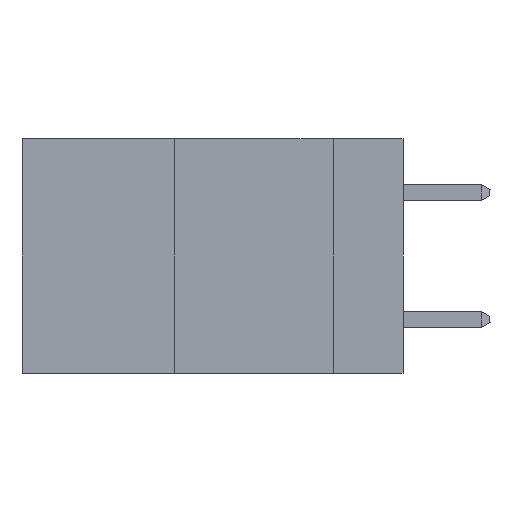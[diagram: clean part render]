
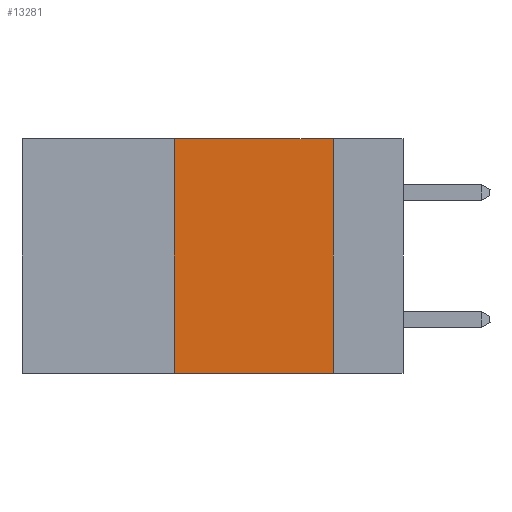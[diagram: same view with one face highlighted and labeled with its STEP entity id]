
A CAD part, left-side view. The second image highlights one B-rep face of the part: STEP entity #13281.
In plain terms, the highlighted planar face has unit normal (-1, 0, 0).
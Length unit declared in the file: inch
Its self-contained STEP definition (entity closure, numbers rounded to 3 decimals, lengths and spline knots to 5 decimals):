
#2290 = DIRECTION ( 'NONE',  ( 0., 0., -1. ) ) ;
#2624 = VECTOR ( 'NONE', #29477, 39.37008 ) ;
#3059 = EDGE_CURVE ( 'NONE', #30316, #32605, #28128, .T. ) ;
#5419 = CARTESIAN_POINT ( 'NONE',  ( 0., 0.6, -0.37 ) ) ;
#5584 = LINE ( 'NONE', #10480, #2624 ) ;
#6482 = LINE ( 'NONE', #5419, #34356 ) ;
#6638 = DIRECTION ( 'NONE',  ( 0., 0., 1. ) ) ;
#6868 = CARTESIAN_POINT ( 'NONE',  ( 0., 0.36, 0. ) ) ;
#7020 = EDGE_LOOP ( 'NONE', ( #10697, #21359, #32288, #18349 ) ) ;
#7738 = PLANE ( 'NONE',  #25374 ) ;
#7914 = DIRECTION ( 'NONE',  ( 0., -1., 0. ) ) ;
#9206 = VERTEX_POINT ( 'NONE', #33577 ) ;
#10480 = CARTESIAN_POINT ( 'NONE',  ( 0., 0.6, 0. ) ) ;
#10697 = ORIENTED_EDGE ( 'NONE', *, *, #19433, .F. ) ;
#10961 = LINE ( 'NONE', #13125, #34596 ) ;
#12900 = VECTOR ( 'NONE', #6638, 39.37008 ) ;
#13125 = CARTESIAN_POINT ( 'NONE',  ( 0., 0.11, 0. ) ) ;
#13281 = ADVANCED_FACE ( 'NONE', ( #32293 ), #7738, .F. ) ;
#14251 = EDGE_CURVE ( 'NONE', #32605, #25873, #5584, .T. ) ;
#17828 = CARTESIAN_POINT ( 'NONE',  ( 0., 0.36, 0. ) ) ;
#18349 = ORIENTED_EDGE ( 'NONE', *, *, #22391, .T. ) ;
#19433 = EDGE_CURVE ( 'NONE', #25873, #9206, #10961, .T. ) ;
#21359 = ORIENTED_EDGE ( 'NONE', *, *, #14251, .F. ) ;
#22391 = EDGE_CURVE ( 'NONE', #30316, #9206, #6482, .T. ) ;
#23968 = DIRECTION ( 'NONE',  ( 0., 0., -1. ) ) ;
#24034 = CARTESIAN_POINT ( 'NONE',  ( 0., 0.11, 0. ) ) ;
#25374 = AXIS2_PLACEMENT_3D ( 'NONE', #26528, #32184, #2290 ) ;
#25873 = VERTEX_POINT ( 'NONE', #24034 ) ;
#26528 = CARTESIAN_POINT ( 'NONE',  ( 0., 0.6, 0. ) ) ;
#28128 = LINE ( 'NONE', #6868, #12900 ) ;
#29477 = DIRECTION ( 'NONE',  ( 0., -1., 0. ) ) ;
#30316 = VERTEX_POINT ( 'NONE', #32462 ) ;
#32184 = DIRECTION ( 'NONE',  ( 1., 0., 0. ) ) ;
#32288 = ORIENTED_EDGE ( 'NONE', *, *, #3059, .F. ) ;
#32293 = FACE_OUTER_BOUND ( 'NONE', #7020, .T. ) ;
#32462 = CARTESIAN_POINT ( 'NONE',  ( 0., 0.36, -0.37 ) ) ;
#32605 = VERTEX_POINT ( 'NONE', #17828 ) ;
#33577 = CARTESIAN_POINT ( 'NONE',  ( 0., 0.11, -0.37 ) ) ;
#34356 = VECTOR ( 'NONE', #7914, 39.37008 ) ;
#34596 = VECTOR ( 'NONE', #23968, 39.37008 ) ;
